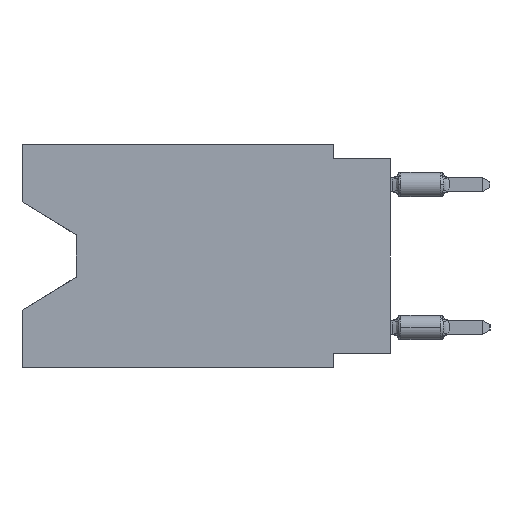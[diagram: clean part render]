
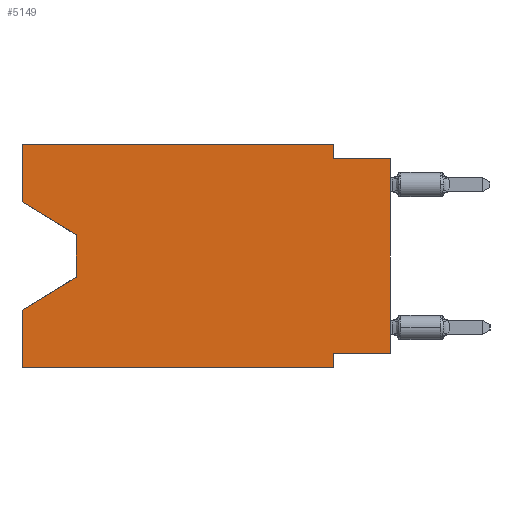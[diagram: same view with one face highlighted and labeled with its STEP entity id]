
A CAD part, left-side view. The second image highlights one B-rep face of the part: STEP entity #5149.
In plain terms, the highlighted planar face has unit normal (-1, 0, 0).
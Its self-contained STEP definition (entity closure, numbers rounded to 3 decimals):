
#462 = EDGE_CURVE ( 'NONE', #27820, #4557, #25511, .T. ) ;
#876 = FACE_OUTER_BOUND ( 'NONE', #7640, .T. ) ;
#1048 = EDGE_CURVE ( 'NONE', #14952, #26289, #29566, .T. ) ;
#1392 = VECTOR ( 'NONE', #28480, 1000. ) ;
#1557 = EDGE_CURVE ( 'NONE', #31620, #23789, #4544, .T. ) ;
#1644 = CARTESIAN_POINT ( 'NONE',  ( 0., 2.54, 0. ) ) ;
#2086 = DIRECTION ( 'NONE',  ( 0., -1., 0. ) ) ;
#2498 = ORIENTED_EDGE ( 'NONE', *, *, #5815, .T. ) ;
#3522 = VECTOR ( 'NONE', #2086, 1000. ) ;
#3997 = ORIENTED_EDGE ( 'NONE', *, *, #10070, .T. ) ;
#4173 = CARTESIAN_POINT ( 'NONE',  ( 0., 16.383, -2.546 ) ) ;
#4544 = LINE ( 'NONE', #6600, #13693 ) ;
#4557 = VERTEX_POINT ( 'NONE', #35300 ) ;
#4976 = CARTESIAN_POINT ( 'NONE',  ( 0., 0., -9.271 ) ) ;
#5149 = ADVANCED_FACE ( 'NONE', ( #876 ), #11786, .F. ) ;
#5191 = ORIENTED_EDGE ( 'NONE', *, *, #1557, .T. ) ;
#5288 = ORIENTED_EDGE ( 'NONE', *, *, #1048, .F. ) ;
#5722 = DIRECTION ( 'NONE',  ( 0., 0., 1. ) ) ;
#5815 = EDGE_CURVE ( 'NONE', #19602, #26289, #6718, .T. ) ;
#6600 = CARTESIAN_POINT ( 'NONE',  ( 0., 13.97, -5.893 ) ) ;
#6718 = LINE ( 'NONE', #33752, #16839 ) ;
#7005 = CARTESIAN_POINT ( 'NONE',  ( 0., 16.383, -2.546 ) ) ;
#7310 = LINE ( 'NONE', #21634, #29976 ) ;
#7640 = EDGE_LOOP ( 'NONE', ( #12878, #3997, #5191, #23769, #2498, #5288, #12926, #19960, #25679, #29697, #31582, #7673 ) ) ;
#7673 = ORIENTED_EDGE ( 'NONE', *, *, #13681, .F. ) ;
#8562 = EDGE_CURVE ( 'NONE', #28667, #14579, #26625, .T. ) ;
#8871 = DIRECTION ( 'NONE',  ( 0., -1., 0. ) ) ;
#9608 = EDGE_CURVE ( 'NONE', #29285, #28667, #23326, .T. ) ;
#9885 = VECTOR ( 'NONE', #18195, 1000. ) ;
#10070 = EDGE_CURVE ( 'NONE', #4557, #31620, #28623, .T. ) ;
#10663 = CARTESIAN_POINT ( 'NONE',  ( 0., 16.383, -9.906 ) ) ;
#11266 = LINE ( 'NONE', #16279, #26456 ) ;
#11786 = PLANE ( 'NONE',  #32023 ) ;
#12118 = DIRECTION ( 'NONE',  ( 0., 0.855, -0.519 ) ) ;
#12659 = DIRECTION ( 'NONE',  ( 0., 1., 0. ) ) ;
#12878 = ORIENTED_EDGE ( 'NONE', *, *, #462, .T. ) ;
#12926 = ORIENTED_EDGE ( 'NONE', *, *, #30776, .F. ) ;
#13681 = EDGE_CURVE ( 'NONE', #27820, #21436, #11266, .T. ) ;
#13693 = VECTOR ( 'NONE', #12118, 1000. ) ;
#14579 = VERTEX_POINT ( 'NONE', #32510 ) ;
#14790 = VECTOR ( 'NONE', #31242, 1000. ) ;
#14952 = VERTEX_POINT ( 'NONE', #29607 ) ;
#15682 = CARTESIAN_POINT ( 'NONE',  ( 0., 16.383, 0. ) ) ;
#15701 = LINE ( 'NONE', #4976, #27806 ) ;
#16279 = CARTESIAN_POINT ( 'NONE',  ( 0., 16.383, 0. ) ) ;
#16839 = VECTOR ( 'NONE', #8871, 1000. ) ;
#17700 = EDGE_CURVE ( 'NONE', #19602, #23789, #24364, .T. ) ;
#18195 = DIRECTION ( 'NONE',  ( 0., 0., -1. ) ) ;
#18282 = EDGE_CURVE ( 'NONE', #21436, #29285, #28954, .T. ) ;
#18441 = DIRECTION ( 'NONE',  ( 0., 0., -1. ) ) ;
#19602 = VERTEX_POINT ( 'NONE', #10663 ) ;
#19674 = DIRECTION ( 'NONE',  ( 1., 0., 0. ) ) ;
#19908 = CARTESIAN_POINT ( 'NONE',  ( 0., 16.383, -7.36 ) ) ;
#19960 = ORIENTED_EDGE ( 'NONE', *, *, #28321, .T. ) ;
#20015 = CARTESIAN_POINT ( 'NONE',  ( 0., 16.383, 0. ) ) ;
#21008 = CARTESIAN_POINT ( 'NONE',  ( 0., 13.97, -5.893 ) ) ;
#21436 = VERTEX_POINT ( 'NONE', #15682 ) ;
#21634 = CARTESIAN_POINT ( 'NONE',  ( 0., 0., 0. ) ) ;
#23040 = DIRECTION ( 'NONE',  ( 0., -1., 0. ) ) ;
#23326 = LINE ( 'NONE', #1644, #32514 ) ;
#23769 = ORIENTED_EDGE ( 'NONE', *, *, #17700, .F. ) ;
#23789 = VERTEX_POINT ( 'NONE', #19908 ) ;
#23965 = DIRECTION ( 'NONE',  ( 0., 0., 1. ) ) ;
#24364 = LINE ( 'NONE', #35281, #1392 ) ;
#25511 = LINE ( 'NONE', #4173, #14790 ) ;
#25679 = ORIENTED_EDGE ( 'NONE', *, *, #8562, .F. ) ;
#25893 = CARTESIAN_POINT ( 'NONE',  ( 0., 16.383, 0. ) ) ;
#26289 = VERTEX_POINT ( 'NONE', #27283 ) ;
#26456 = VECTOR ( 'NONE', #5722, 1000. ) ;
#26625 = LINE ( 'NONE', #29128, #3522 ) ;
#27283 = CARTESIAN_POINT ( 'NONE',  ( 0., 2.54, -9.906 ) ) ;
#27806 = VECTOR ( 'NONE', #12659, 1000. ) ;
#27820 = VERTEX_POINT ( 'NONE', #7005 ) ;
#28321 = EDGE_CURVE ( 'NONE', #28505, #14579, #7310, .T. ) ;
#28480 = DIRECTION ( 'NONE',  ( 0., 0., 1. ) ) ;
#28505 = VERTEX_POINT ( 'NONE', #33269 ) ;
#28623 = LINE ( 'NONE', #33985, #9885 ) ;
#28667 = VERTEX_POINT ( 'NONE', #35136 ) ;
#28888 = DIRECTION ( 'NONE',  ( 0., 0., -1. ) ) ;
#28954 = LINE ( 'NONE', #25893, #31721 ) ;
#29128 = CARTESIAN_POINT ( 'NONE',  ( 0., 0., -0.635 ) ) ;
#29285 = VERTEX_POINT ( 'NONE', #30449 ) ;
#29566 = LINE ( 'NONE', #29744, #34249 ) ;
#29607 = CARTESIAN_POINT ( 'NONE',  ( 0., 2.54, -9.271 ) ) ;
#29697 = ORIENTED_EDGE ( 'NONE', *, *, #9608, .F. ) ;
#29744 = CARTESIAN_POINT ( 'NONE',  ( 0., 2.54, -9.906 ) ) ;
#29976 = VECTOR ( 'NONE', #23965, 1000. ) ;
#30449 = CARTESIAN_POINT ( 'NONE',  ( 0., 2.54, 0. ) ) ;
#30776 = EDGE_CURVE ( 'NONE', #28505, #14952, #15701, .T. ) ;
#31242 = DIRECTION ( 'NONE',  ( 0., -0.855, -0.519 ) ) ;
#31582 = ORIENTED_EDGE ( 'NONE', *, *, #18282, .F. ) ;
#31620 = VERTEX_POINT ( 'NONE', #21008 ) ;
#31721 = VECTOR ( 'NONE', #23040, 1000. ) ;
#32023 = AXIS2_PLACEMENT_3D ( 'NONE', #20015, #19674, #33642 ) ;
#32510 = CARTESIAN_POINT ( 'NONE',  ( 0., 0., -0.635 ) ) ;
#32514 = VECTOR ( 'NONE', #28888, 1000. ) ;
#33269 = CARTESIAN_POINT ( 'NONE',  ( 0., 0., -9.271 ) ) ;
#33642 = DIRECTION ( 'NONE',  ( 0., 0., -1. ) ) ;
#33752 = CARTESIAN_POINT ( 'NONE',  ( 0., 16.383, -9.906 ) ) ;
#33985 = CARTESIAN_POINT ( 'NONE',  ( 0., 13.97, -4.013 ) ) ;
#34249 = VECTOR ( 'NONE', #18441, 1000. ) ;
#35136 = CARTESIAN_POINT ( 'NONE',  ( 0., 2.54, -0.635 ) ) ;
#35281 = CARTESIAN_POINT ( 'NONE',  ( 0., 16.383, 0. ) ) ;
#35300 = CARTESIAN_POINT ( 'NONE',  ( 0., 13.97, -4.013 ) ) ;
